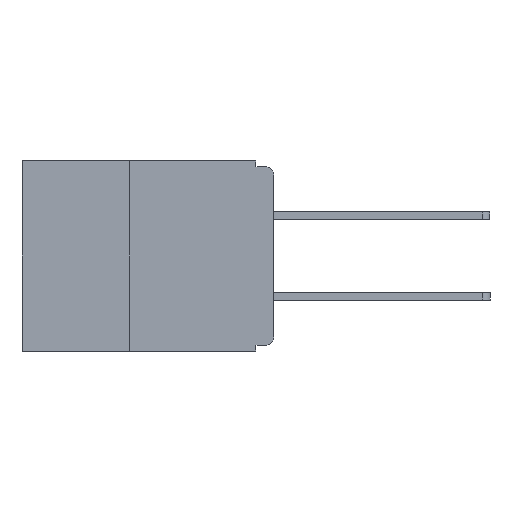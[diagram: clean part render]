
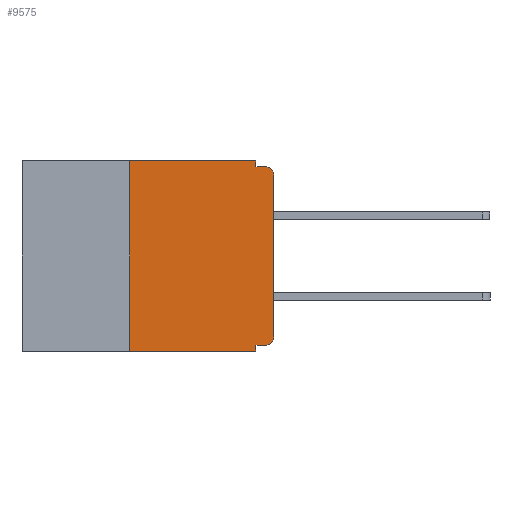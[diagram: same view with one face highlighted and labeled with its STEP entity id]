
A CAD part, left-side view. The second image highlights one B-rep face of the part: STEP entity #9575.
In plain terms, the highlighted planar face has unit normal (-1, 0, 0).
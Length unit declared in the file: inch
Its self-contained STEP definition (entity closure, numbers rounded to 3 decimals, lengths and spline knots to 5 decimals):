
#735 = DIRECTION ( 'NONE',  ( -1., 0., 0. ) ) ;
#1894 = CARTESIAN_POINT ( 'NONE',  ( 0., 0.437, 0. ) ) ;
#2336 = VERTEX_POINT ( 'NONE', #23614 ) ;
#2386 = EDGE_CURVE ( 'NONE', #31916, #30956, #21339, .T. ) ;
#3505 = CARTESIAN_POINT ( 'NONE',  ( 0., 0.031, -0.33 ) ) ;
#4600 = AXIS2_PLACEMENT_3D ( 'NONE', #18224, #18186, #18114 ) ;
#5061 = ORIENTED_EDGE ( 'NONE', *, *, #13737, .F. ) ;
#6170 = CARTESIAN_POINT ( 'NONE',  ( 0., 0.25, -0.33 ) ) ;
#6177 = DIRECTION ( 'NONE',  ( 0., 0., -1. ) ) ;
#6552 = EDGE_CURVE ( 'NONE', #2336, #23531, #14102, .T. ) ;
#7634 = CARTESIAN_POINT ( 'NONE',  ( 0., 0.031, 0. ) ) ;
#9575 = ADVANCED_FACE ( 'NONE', ( #18767 ), #15066, .F. ) ;
#9892 = LINE ( 'NONE', #3505, #22822 ) ;
#11123 = DIRECTION ( 'NONE',  ( 0., 1., 0. ) ) ;
#11189 = DIRECTION ( 'NONE',  ( 0., -1., 0. ) ) ;
#11453 = CARTESIAN_POINT ( 'NONE',  ( 0., 0.25, 0. ) ) ;
#11917 = EDGE_CURVE ( 'NONE', #20959, #27306, #13228, .T. ) ;
#12022 = LINE ( 'NONE', #1894, #30156 ) ;
#12312 = LINE ( 'NONE', #24091, #25259 ) ;
#12629 = ORIENTED_EDGE ( 'NONE', *, *, #28614, .T. ) ;
#12784 = EDGE_CURVE ( 'NONE', #30956, #23531, #20092, .T. ) ;
#12841 = ORIENTED_EDGE ( 'NONE', *, *, #14323, .T. ) ;
#13228 = LINE ( 'NONE', #6170, #26200 ) ;
#13294 = CARTESIAN_POINT ( 'NONE',  ( 0., 0.031, 0. ) ) ;
#13707 = CARTESIAN_POINT ( 'NONE',  ( 0., 0., -0.32 ) ) ;
#13737 = EDGE_CURVE ( 'NONE', #22724, #33583, #9892, .T. ) ;
#13921 = VERTEX_POINT ( 'NONE', #27608 ) ;
#14102 = CIRCLE ( 'NONE', #4600, 0.015 ) ;
#14323 = EDGE_CURVE ( 'NONE', #20959, #33583, #12312, .T. ) ;
#14467 = VECTOR ( 'NONE', #21343, 39.37008 ) ;
#14998 = DIRECTION ( 'NONE',  ( 0., 0., -1. ) ) ;
#15031 = DIRECTION ( 'NONE',  ( 1., 0., 0. ) ) ;
#15066 = PLANE ( 'NONE',  #20837 ) ;
#15224 = CARTESIAN_POINT ( 'NONE',  ( 0., 0.437, 0. ) ) ;
#16221 = VECTOR ( 'NONE', #11123, 39.37008 ) ;
#16379 = EDGE_CURVE ( 'NONE', #13921, #22724, #17063, .T. ) ;
#16488 = CARTESIAN_POINT ( 'NONE',  ( 0., 0.015, -0.305 ) ) ;
#16551 = DIRECTION ( 'NONE',  ( 0., 0., 1. ) ) ;
#17063 = LINE ( 'NONE', #13707, #16221 ) ;
#17416 = CARTESIAN_POINT ( 'NONE',  ( 0., 0., -0.01 ) ) ;
#18114 = DIRECTION ( 'NONE',  ( 0., 0., -1. ) ) ;
#18186 = DIRECTION ( 'NONE',  ( -1., 0., 0. ) ) ;
#18224 = CARTESIAN_POINT ( 'NONE',  ( 0., 0.015, -0.025 ) ) ;
#18408 = EDGE_CURVE ( 'NONE', #13921, #18986, #24746, .T. ) ;
#18767 = FACE_OUTER_BOUND ( 'NONE', #31399, .T. ) ;
#18986 = VERTEX_POINT ( 'NONE', #21181 ) ;
#19098 = DIRECTION ( 'NONE',  ( 0., 0., -1. ) ) ;
#19173 = ORIENTED_EDGE ( 'NONE', *, *, #18408, .T. ) ;
#19530 = DIRECTION ( 'NONE',  ( 0., 0., 1. ) ) ;
#20092 = LINE ( 'NONE', #17416, #32086 ) ;
#20760 = CARTESIAN_POINT ( 'NONE',  ( 0., 0.25, -0.33 ) ) ;
#20831 = EDGE_CURVE ( 'NONE', #27306, #31916, #12022, .T. ) ;
#20837 = AXIS2_PLACEMENT_3D ( 'NONE', #15224, #15031, #14998 ) ;
#20959 = VERTEX_POINT ( 'NONE', #20760 ) ;
#21181 = CARTESIAN_POINT ( 'NONE',  ( 0., 0., -0.305 ) ) ;
#21339 = LINE ( 'NONE', #7634, #14467 ) ;
#21343 = DIRECTION ( 'NONE',  ( 0., 0., -1. ) ) ;
#21503 = ORIENTED_EDGE ( 'NONE', *, *, #11917, .F. ) ;
#22564 = ORIENTED_EDGE ( 'NONE', *, *, #6552, .T. ) ;
#22672 = CARTESIAN_POINT ( 'NONE',  ( 0., 0.031, -0.32 ) ) ;
#22724 = VERTEX_POINT ( 'NONE', #22672 ) ;
#22786 = DIRECTION ( 'NONE',  ( 0., -1., 0. ) ) ;
#22822 = VECTOR ( 'NONE', #6177, 39.37008 ) ;
#23531 = VERTEX_POINT ( 'NONE', #27193 ) ;
#23614 = CARTESIAN_POINT ( 'NONE',  ( 0., 0., -0.025 ) ) ;
#23767 = ORIENTED_EDGE ( 'NONE', *, *, #16379, .F. ) ;
#24091 = CARTESIAN_POINT ( 'NONE',  ( 0., 0.437, -0.33 ) ) ;
#24325 = AXIS2_PLACEMENT_3D ( 'NONE', #16488, #735, #19098 ) ;
#24746 = CIRCLE ( 'NONE', #24325, 0.015 ) ;
#25259 = VECTOR ( 'NONE', #11189, 39.37008 ) ;
#25376 = ORIENTED_EDGE ( 'NONE', *, *, #2386, .F. ) ;
#25415 = CARTESIAN_POINT ( 'NONE',  ( 0., 0.031, -0.33 ) ) ;
#26200 = VECTOR ( 'NONE', #16551, 39.37008 ) ;
#26518 = ORIENTED_EDGE ( 'NONE', *, *, #12784, .F. ) ;
#27193 = CARTESIAN_POINT ( 'NONE',  ( 0., 0.015, -0.01 ) ) ;
#27306 = VERTEX_POINT ( 'NONE', #11453 ) ;
#27608 = CARTESIAN_POINT ( 'NONE',  ( 0., 0.015, -0.32 ) ) ;
#27771 = DIRECTION ( 'NONE',  ( 0., -1., 0. ) ) ;
#28614 = EDGE_CURVE ( 'NONE', #18986, #2336, #32587, .T. ) ;
#30156 = VECTOR ( 'NONE', #22786, 39.37008 ) ;
#30225 = VECTOR ( 'NONE', #19530, 39.37008 ) ;
#30556 = CARTESIAN_POINT ( 'NONE',  ( 0., 0.031, -0.01 ) ) ;
#30956 = VERTEX_POINT ( 'NONE', #30556 ) ;
#31399 = EDGE_LOOP ( 'NONE', ( #12629, #22564, #26518, #25376, #31494, #21503, #12841, #5061, #23767, #19173 ) ) ;
#31494 = ORIENTED_EDGE ( 'NONE', *, *, #20831, .F. ) ;
#31916 = VERTEX_POINT ( 'NONE', #13294 ) ;
#32086 = VECTOR ( 'NONE', #27771, 39.37008 ) ;
#32267 = CARTESIAN_POINT ( 'NONE',  ( 0., 0., 0. ) ) ;
#32587 = LINE ( 'NONE', #32267, #30225 ) ;
#33583 = VERTEX_POINT ( 'NONE', #25415 ) ;
